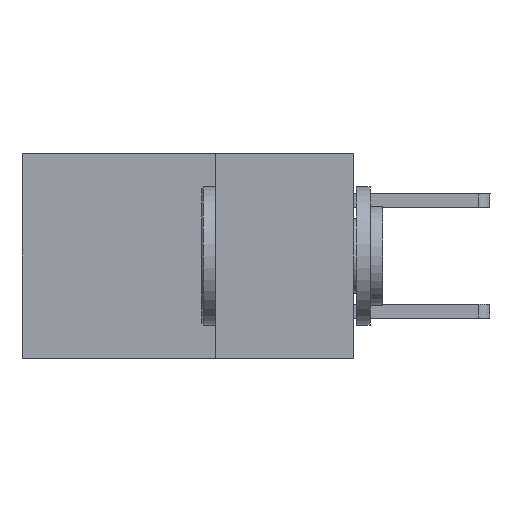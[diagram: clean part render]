
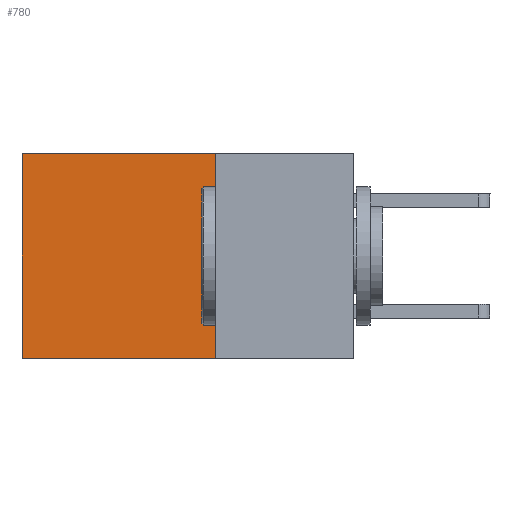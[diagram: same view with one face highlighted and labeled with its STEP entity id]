
A CAD part, left-side view. The second image highlights one B-rep face of the part: STEP entity #780.
In plain terms, the highlighted planar face has unit normal (-1, 0, 0).
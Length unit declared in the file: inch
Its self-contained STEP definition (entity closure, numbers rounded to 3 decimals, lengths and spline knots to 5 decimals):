
#356 = DIRECTION ( 'NONE',  ( 0., 1., 0. ) ) ;
#369 = AXIS2_PLACEMENT_3D ( 'NONE', #9117, #744, #647 ) ;
#593 = ORIENTED_EDGE ( 'NONE', *, *, #10092, .T. ) ;
#647 = DIRECTION ( 'NONE',  ( 0., 0., -1. ) ) ;
#744 = DIRECTION ( 'NONE',  ( 1., 0., 0. ) ) ;
#780 = ADVANCED_FACE ( 'NONE', ( #4063 ), #3392, .F. ) ;
#1482 = VERTEX_POINT ( 'NONE', #8944 ) ;
#1897 = VECTOR ( 'NONE', #3745, 39.37008 ) ;
#2370 = EDGE_CURVE ( 'NONE', #9712, #1482, #7448, .T. ) ;
#2552 = LINE ( 'NONE', #8511, #1897 ) ;
#2757 = LINE ( 'NONE', #6538, #8842 ) ;
#2941 = CARTESIAN_POINT ( 'NONE',  ( 0.2875, 0.6, 0. ) ) ;
#2980 = VECTOR ( 'NONE', #6876, 39.37008 ) ;
#3093 = ORIENTED_EDGE ( 'NONE', *, *, #2370, .F. ) ;
#3392 = PLANE ( 'NONE',  #369 ) ;
#3745 = DIRECTION ( 'NONE',  ( 0., 0., -1. ) ) ;
#4063 = FACE_OUTER_BOUND ( 'NONE', #7884, .T. ) ;
#5672 = LINE ( 'NONE', #2941, #2980 ) ;
#6081 = CARTESIAN_POINT ( 'NONE',  ( 0.2875, 0.25, -0.37 ) ) ;
#6538 = CARTESIAN_POINT ( 'NONE',  ( 0.2875, 0.25, 0. ) ) ;
#6876 = DIRECTION ( 'NONE',  ( 0., 0., -1. ) ) ;
#7362 = CARTESIAN_POINT ( 'NONE',  ( 0.2875, 0.6, 0. ) ) ;
#7448 = LINE ( 'NONE', #10482, #9722 ) ;
#7860 = EDGE_CURVE ( 'NONE', #10740, #1482, #5672, .T. ) ;
#7884 = EDGE_LOOP ( 'NONE', ( #12665, #3093, #10783, #593 ) ) ;
#8303 = VERTEX_POINT ( 'NONE', #9273 ) ;
#8511 = CARTESIAN_POINT ( 'NONE',  ( 0.2875, 0.25, 0. ) ) ;
#8842 = VECTOR ( 'NONE', #356, 39.37008 ) ;
#8944 = CARTESIAN_POINT ( 'NONE',  ( 0.2875, 0.6, -0.37 ) ) ;
#9117 = CARTESIAN_POINT ( 'NONE',  ( 0.2875, 0.25, 0. ) ) ;
#9273 = CARTESIAN_POINT ( 'NONE',  ( 0.2875, 0.25, 0. ) ) ;
#9712 = VERTEX_POINT ( 'NONE', #6081 ) ;
#9722 = VECTOR ( 'NONE', #9952, 39.37008 ) ;
#9952 = DIRECTION ( 'NONE',  ( 0., 1., 0. ) ) ;
#10092 = EDGE_CURVE ( 'NONE', #8303, #10740, #2757, .T. ) ;
#10482 = CARTESIAN_POINT ( 'NONE',  ( 0.2875, 0.25, -0.37 ) ) ;
#10740 = VERTEX_POINT ( 'NONE', #7362 ) ;
#10783 = ORIENTED_EDGE ( 'NONE', *, *, #10900, .F. ) ;
#10900 = EDGE_CURVE ( 'NONE', #8303, #9712, #2552, .T. ) ;
#12665 = ORIENTED_EDGE ( 'NONE', *, *, #7860, .T. ) ;
